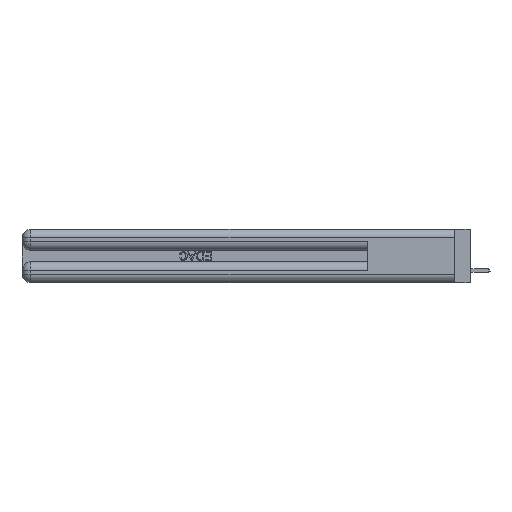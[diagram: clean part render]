
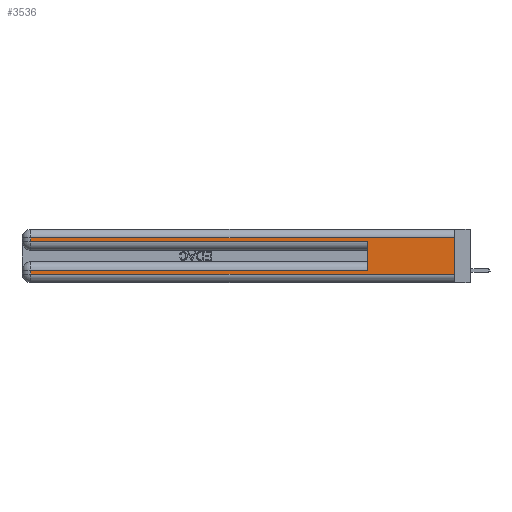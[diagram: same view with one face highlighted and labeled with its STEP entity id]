
A CAD part, left-side view. The second image highlights one B-rep face of the part: STEP entity #3536.
In plain terms, the highlighted planar face has unit normal (-1, 0, 0).
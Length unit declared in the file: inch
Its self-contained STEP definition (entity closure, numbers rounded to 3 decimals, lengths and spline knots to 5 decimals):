
#177 = ORIENTED_EDGE ( 'NONE', *, *, #21136, .T. ) ;
#202 = VERTEX_POINT ( 'NONE', #8312 ) ;
#360 = LINE ( 'NONE', #28093, #5275 ) ;
#661 = VERTEX_POINT ( 'NONE', #26433 ) ;
#734 = VERTEX_POINT ( 'NONE', #29824 ) ;
#896 = VECTOR ( 'NONE', #25166, 39.37008 ) ;
#1510 = LINE ( 'NONE', #48511, #896 ) ;
#3358 = VECTOR ( 'NONE', #48214, 39.37008 ) ;
#3536 = ADVANCED_FACE ( 'NONE', ( #13749 ), #29478, .F. ) ;
#4324 = VERTEX_POINT ( 'NONE', #10020 ) ;
#4994 = CARTESIAN_POINT ( 'NONE',  ( 0., 0., 0.37 ) ) ;
#5275 = VECTOR ( 'NONE', #48212, 39.37008 ) ;
#5778 = LINE ( 'NONE', #20943, #3358 ) ;
#7219 = LINE ( 'NONE', #19747, #18194 ) ;
#8312 = CARTESIAN_POINT ( 'NONE',  ( 0., 2.94, 0.31 ) ) ;
#8791 = DIRECTION ( 'NONE',  ( 0., 0., -1. ) ) ;
#10020 = CARTESIAN_POINT ( 'NONE',  ( 0., 2.94, 0.085 ) ) ;
#11334 = AXIS2_PLACEMENT_3D ( 'NONE', #4994, #17131, #8791 ) ;
#12063 = CARTESIAN_POINT ( 'NONE',  ( 0., 0., 0.31 ) ) ;
#12175 = VERTEX_POINT ( 'NONE', #14971 ) ;
#12337 = EDGE_CURVE ( 'NONE', #16619, #661, #41292, .T. ) ;
#13178 = CARTESIAN_POINT ( 'NONE',  ( 0., 0., 0.06 ) ) ;
#13234 = LINE ( 'NONE', #28360, #19394 ) ;
#13550 = EDGE_LOOP ( 'NONE', ( #18533, #27314, #16652, #177, #42400, #27852, #43024, #24559 ) ) ;
#13749 = FACE_OUTER_BOUND ( 'NONE', #13550, .T. ) ;
#14971 = CARTESIAN_POINT ( 'NONE',  ( 0., 0.6, 0.085 ) ) ;
#15689 = DIRECTION ( 'NONE',  ( 0., 0., -1. ) ) ;
#16619 = VERTEX_POINT ( 'NONE', #44559 ) ;
#16652 = ORIENTED_EDGE ( 'NONE', *, *, #48910, .T. ) ;
#17131 = DIRECTION ( 'NONE',  ( 1., 0., 0. ) ) ;
#18194 = VECTOR ( 'NONE', #15689, 39.37008 ) ;
#18533 = ORIENTED_EDGE ( 'NONE', *, *, #12337, .F. ) ;
#19394 = VECTOR ( 'NONE', #24628, 39.37008 ) ;
#19747 = CARTESIAN_POINT ( 'NONE',  ( 0., 2.94, 0.37 ) ) ;
#20617 = EDGE_CURVE ( 'NONE', #12175, #4324, #360, .T. ) ;
#20943 = CARTESIAN_POINT ( 'NONE',  ( 0., 2.94, 0.37 ) ) ;
#21136 = EDGE_CURVE ( 'NONE', #31390, #39870, #1510, .T. ) ;
#22664 = DIRECTION ( 'NONE',  ( 0., 0., -1. ) ) ;
#23372 = DIRECTION ( 'NONE',  ( 0., 1., 0. ) ) ;
#24559 = ORIENTED_EDGE ( 'NONE', *, *, #46129, .T. ) ;
#24628 = DIRECTION ( 'NONE',  ( 0., 0., 1. ) ) ;
#25166 = DIRECTION ( 'NONE',  ( 0., -1., 0. ) ) ;
#25652 = CARTESIAN_POINT ( 'NONE',  ( 0., 0.6, 0.285 ) ) ;
#26375 = VECTOR ( 'NONE', #44391, 39.37008 ) ;
#26433 = CARTESIAN_POINT ( 'NONE',  ( 0., 0., 0.06 ) ) ;
#27314 = ORIENTED_EDGE ( 'NONE', *, *, #31563, .T. ) ;
#27852 = ORIENTED_EDGE ( 'NONE', *, *, #20617, .T. ) ;
#28093 = CARTESIAN_POINT ( 'NONE',  ( 0., 0., 0.085 ) ) ;
#28360 = CARTESIAN_POINT ( 'NONE',  ( 0., 0.6, 0.145 ) ) ;
#29081 = EDGE_CURVE ( 'NONE', #4324, #734, #5778, .T. ) ;
#29478 = PLANE ( 'NONE',  #11334 ) ;
#29824 = CARTESIAN_POINT ( 'NONE',  ( 0., 2.94, 0.06 ) ) ;
#31390 = VERTEX_POINT ( 'NONE', #50205 ) ;
#31563 = EDGE_CURVE ( 'NONE', #16619, #202, #46574, .T. ) ;
#36068 = VECTOR ( 'NONE', #23372, 39.37008 ) ;
#36635 = LINE ( 'NONE', #13178, #26375 ) ;
#39870 = VERTEX_POINT ( 'NONE', #25652 ) ;
#41292 = LINE ( 'NONE', #46006, #47946 ) ;
#42400 = ORIENTED_EDGE ( 'NONE', *, *, #43175, .F. ) ;
#43024 = ORIENTED_EDGE ( 'NONE', *, *, #29081, .T. ) ;
#43175 = EDGE_CURVE ( 'NONE', #12175, #39870, #13234, .T. ) ;
#44391 = DIRECTION ( 'NONE',  ( 0., -1., 0. ) ) ;
#44559 = CARTESIAN_POINT ( 'NONE',  ( 0., 0., 0.31 ) ) ;
#46006 = CARTESIAN_POINT ( 'NONE',  ( 0., 0., 0.37 ) ) ;
#46129 = EDGE_CURVE ( 'NONE', #734, #661, #36635, .T. ) ;
#46574 = LINE ( 'NONE', #12063, #36068 ) ;
#47946 = VECTOR ( 'NONE', #22664, 39.37008 ) ;
#48212 = DIRECTION ( 'NONE',  ( 0., 1., 0. ) ) ;
#48214 = DIRECTION ( 'NONE',  ( 0., 0., -1. ) ) ;
#48511 = CARTESIAN_POINT ( 'NONE',  ( 0., 0., 0.285 ) ) ;
#48910 = EDGE_CURVE ( 'NONE', #202, #31390, #7219, .T. ) ;
#50205 = CARTESIAN_POINT ( 'NONE',  ( 0., 2.94, 0.285 ) ) ;
